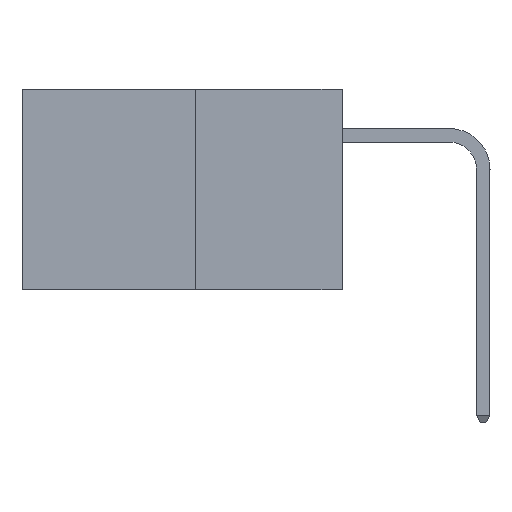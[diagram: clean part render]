
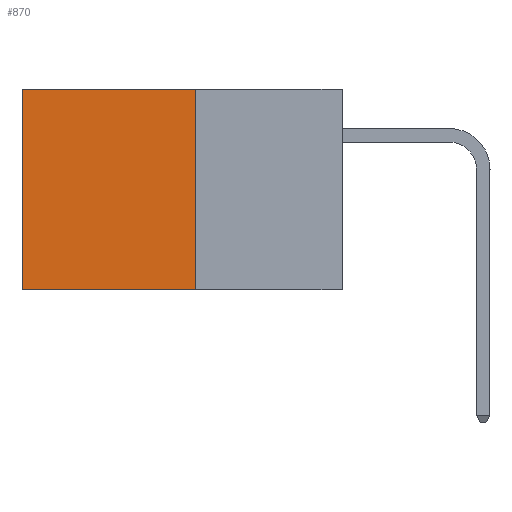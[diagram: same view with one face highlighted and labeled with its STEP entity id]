
A CAD part, left-side view. The second image highlights one B-rep face of the part: STEP entity #870.
In plain terms, the highlighted planar face has unit normal (-1, 0, 0).
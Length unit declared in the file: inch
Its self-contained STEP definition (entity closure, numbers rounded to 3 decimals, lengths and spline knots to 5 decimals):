
#643 = VECTOR ( 'NONE', #18362, 39.37008 ) ;
#802 = CARTESIAN_POINT ( 'NONE',  ( 0.277, 0.59, -0.37 ) ) ;
#870 = ADVANCED_FACE ( 'NONE', ( #5742 ), #5114, .F. ) ;
#2369 = CARTESIAN_POINT ( 'NONE',  ( 0.277, 0.27, -0.37 ) ) ;
#2652 = DIRECTION ( 'NONE',  ( 0., 0., -1. ) ) ;
#2803 = ORIENTED_EDGE ( 'NONE', *, *, #12212, .T. ) ;
#3487 = EDGE_LOOP ( 'NONE', ( #8283, #21466, #9628, #2803 ) ) ;
#4474 = LINE ( 'NONE', #802, #13881 ) ;
#5114 = PLANE ( 'NONE',  #11293 ) ;
#5180 = VERTEX_POINT ( 'NONE', #5637 ) ;
#5637 = CARTESIAN_POINT ( 'NONE',  ( 0.277, 0.59, -0.37 ) ) ;
#5742 = FACE_OUTER_BOUND ( 'NONE', #3487, .T. ) ;
#6328 = CARTESIAN_POINT ( 'NONE',  ( 0.277, 0.27, -0.37 ) ) ;
#7057 = VERTEX_POINT ( 'NONE', #8922 ) ;
#7659 = CARTESIAN_POINT ( 'NONE',  ( 0.277, 0.27, -0.37 ) ) ;
#8082 = DIRECTION ( 'NONE',  ( 0., 1., 0. ) ) ;
#8283 = ORIENTED_EDGE ( 'NONE', *, *, #11406, .T. ) ;
#8922 = CARTESIAN_POINT ( 'NONE',  ( 0.277, 0.59, 0. ) ) ;
#9396 = DIRECTION ( 'NONE',  ( 0., 0., -1. ) ) ;
#9628 = ORIENTED_EDGE ( 'NONE', *, *, #20751, .F. ) ;
#9971 = VECTOR ( 'NONE', #19427, 39.37008 ) ;
#10923 = CARTESIAN_POINT ( 'NONE',  ( 0.277, 0.27, 0. ) ) ;
#11293 = AXIS2_PLACEMENT_3D ( 'NONE', #2369, #15451, #9396 ) ;
#11406 = EDGE_CURVE ( 'NONE', #7057, #5180, #4474, .T. ) ;
#12212 = EDGE_CURVE ( 'NONE', #20867, #7057, #14953, .T. ) ;
#12964 = VERTEX_POINT ( 'NONE', #7659 ) ;
#13095 = EDGE_CURVE ( 'NONE', #12964, #5180, #19055, .T. ) ;
#13881 = VECTOR ( 'NONE', #2652, 39.37008 ) ;
#14953 = LINE ( 'NONE', #10923, #643 ) ;
#15451 = DIRECTION ( 'NONE',  ( 1., 0., 0. ) ) ;
#15543 = CARTESIAN_POINT ( 'NONE',  ( 0.277, 0.27, -0.37 ) ) ;
#15926 = CARTESIAN_POINT ( 'NONE',  ( 0.277, 0.27, 0. ) ) ;
#18362 = DIRECTION ( 'NONE',  ( 0., 1., 0. ) ) ;
#19055 = LINE ( 'NONE', #15543, #23435 ) ;
#19334 = LINE ( 'NONE', #6328, #9971 ) ;
#19427 = DIRECTION ( 'NONE',  ( 0., 0., -1. ) ) ;
#20751 = EDGE_CURVE ( 'NONE', #20867, #12964, #19334, .T. ) ;
#20867 = VERTEX_POINT ( 'NONE', #15926 ) ;
#21466 = ORIENTED_EDGE ( 'NONE', *, *, #13095, .F. ) ;
#23435 = VECTOR ( 'NONE', #8082, 39.37008 ) ;
